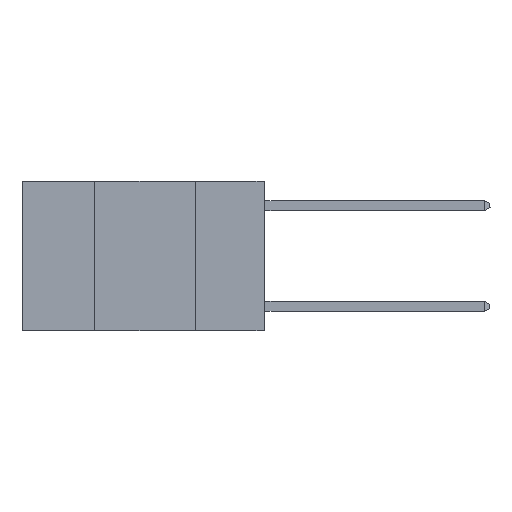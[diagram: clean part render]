
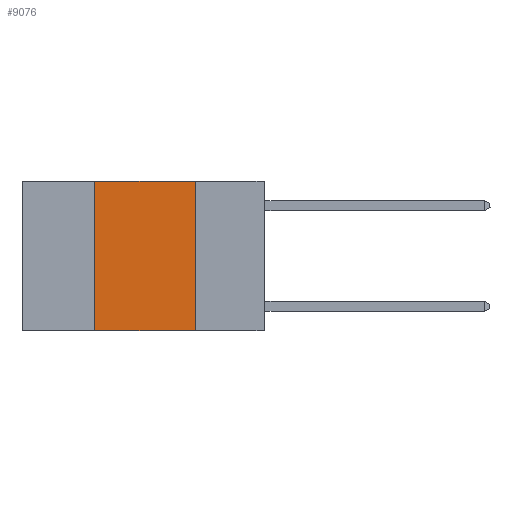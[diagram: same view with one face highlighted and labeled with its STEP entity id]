
A CAD part, left-side view. The second image highlights one B-rep face of the part: STEP entity #9076.
In plain terms, the highlighted planar face has unit normal (-1, 0, 0).
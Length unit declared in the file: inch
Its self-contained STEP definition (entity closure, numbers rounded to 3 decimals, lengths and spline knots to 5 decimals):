
#156 = CARTESIAN_POINT ( 'NONE',  ( 0., 0.42, 0. ) ) ;
#948 = ORIENTED_EDGE ( 'NONE', *, *, #8971, .F. ) ;
#1182 = CARTESIAN_POINT ( 'NONE',  ( 0., 0.17, 0. ) ) ;
#1408 = EDGE_CURVE ( 'NONE', #4265, #2824, #7599, .T. ) ;
#1470 = CARTESIAN_POINT ( 'NONE',  ( 0., 0.6, 0. ) ) ;
#1561 = CARTESIAN_POINT ( 'NONE',  ( 0., 0.17, -0.37 ) ) ;
#1990 = VECTOR ( 'NONE', #9097, 39.37008 ) ;
#2549 = ORIENTED_EDGE ( 'NONE', *, *, #5673, .F. ) ;
#2624 = DIRECTION ( 'NONE',  ( 0., 0., -1. ) ) ;
#2686 = LINE ( 'NONE', #9232, #6260 ) ;
#2801 = ORIENTED_EDGE ( 'NONE', *, *, #6669, .T. ) ;
#2824 = VERTEX_POINT ( 'NONE', #156 ) ;
#2901 = PLANE ( 'NONE',  #5468 ) ;
#3094 = EDGE_LOOP ( 'NONE', ( #948, #2549, #6356, #2801 ) ) ;
#3589 = DIRECTION ( 'NONE',  ( 0., 0., -1. ) ) ;
#4265 = VERTEX_POINT ( 'NONE', #7675 ) ;
#4542 = LINE ( 'NONE', #1182, #8020 ) ;
#4721 = VECTOR ( 'NONE', #8600, 39.37008 ) ;
#4926 = LINE ( 'NONE', #7858, #4721 ) ;
#4955 = DIRECTION ( 'NONE',  ( 0., -1., 0. ) ) ;
#5468 = AXIS2_PLACEMENT_3D ( 'NONE', #1470, #7803, #3589 ) ;
#5673 = EDGE_CURVE ( 'NONE', #2824, #6560, #2686, .T. ) ;
#6260 = VECTOR ( 'NONE', #4955, 39.37008 ) ;
#6313 = FACE_OUTER_BOUND ( 'NONE', #3094, .T. ) ;
#6356 = ORIENTED_EDGE ( 'NONE', *, *, #1408, .F. ) ;
#6560 = VERTEX_POINT ( 'NONE', #7792 ) ;
#6669 = EDGE_CURVE ( 'NONE', #4265, #8573, #4926, .T. ) ;
#7599 = LINE ( 'NONE', #7756, #1990 ) ;
#7675 = CARTESIAN_POINT ( 'NONE',  ( 0., 0.42, -0.37 ) ) ;
#7756 = CARTESIAN_POINT ( 'NONE',  ( 0., 0.42, 0. ) ) ;
#7792 = CARTESIAN_POINT ( 'NONE',  ( 0., 0.17, 0. ) ) ;
#7803 = DIRECTION ( 'NONE',  ( 1., 0., 0. ) ) ;
#7858 = CARTESIAN_POINT ( 'NONE',  ( 0., 0.6, -0.37 ) ) ;
#8020 = VECTOR ( 'NONE', #2624, 39.37008 ) ;
#8573 = VERTEX_POINT ( 'NONE', #1561 ) ;
#8600 = DIRECTION ( 'NONE',  ( 0., -1., 0. ) ) ;
#8971 = EDGE_CURVE ( 'NONE', #6560, #8573, #4542, .T. ) ;
#9076 = ADVANCED_FACE ( 'NONE', ( #6313 ), #2901, .F. ) ;
#9097 = DIRECTION ( 'NONE',  ( 0., 0., 1. ) ) ;
#9232 = CARTESIAN_POINT ( 'NONE',  ( 0., 0.6, 0. ) ) ;
